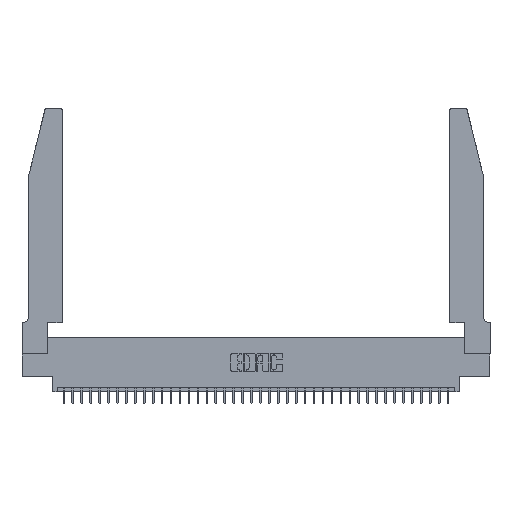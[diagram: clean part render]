
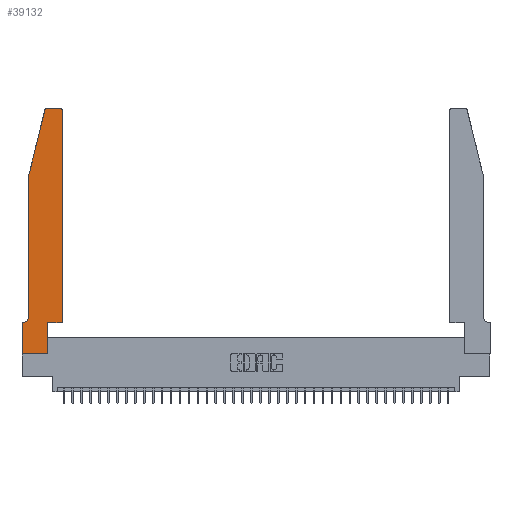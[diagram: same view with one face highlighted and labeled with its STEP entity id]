
A CAD part, top view. The second image highlights one B-rep face of the part: STEP entity #39132.
In plain terms, the highlighted planar face has unit normal (0, 0, 1).
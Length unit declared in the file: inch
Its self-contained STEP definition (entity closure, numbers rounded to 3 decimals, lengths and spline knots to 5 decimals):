
#134 = VERTEX_POINT ( 'NONE', #5959 ) ;
#214 = LINE ( 'NONE', #12319, #29151 ) ;
#238 = CARTESIAN_POINT ( 'NONE',  ( 0.4505, 0.35, 0.37 ) ) ;
#359 = ORIENTED_EDGE ( 'NONE', *, *, #4177, .T. ) ;
#450 = ORIENTED_EDGE ( 'NONE', *, *, #17238, .T. ) ;
#1116 = VECTOR ( 'NONE', #9375, 39.37008 ) ;
#1347 = DIRECTION ( 'NONE',  ( 1., 0., 0. ) ) ;
#1585 = AXIS2_PLACEMENT_3D ( 'NONE', #24656, #33210, #23868 ) ;
#1913 = CARTESIAN_POINT ( 'NONE',  ( 0.2865, 0.35, 0.37 ) ) ;
#2260 = DIRECTION ( 'NONE',  ( -1., 0., 0. ) ) ;
#3173 = LINE ( 'NONE', #27199, #30112 ) ;
#4101 = DIRECTION ( 'NONE',  ( 0., 0., 1. ) ) ;
#4177 = EDGE_CURVE ( 'NONE', #26298, #17205, #36339, .T. ) ;
#4184 = LINE ( 'NONE', #6785, #25889 ) ;
#4280 = CARTESIAN_POINT ( 'NONE',  ( 0., 0., 0.37 ) ) ;
#4679 = ORIENTED_EDGE ( 'NONE', *, *, #5026, .T. ) ;
#4870 = CARTESIAN_POINT ( 'NONE',  ( 0.25487, 2.72718, 0.37 ) ) ;
#5026 = EDGE_CURVE ( 'NONE', #14524, #21064, #29655, .T. ) ;
#5142 = EDGE_CURVE ( 'NONE', #17487, #14524, #12159, .T. ) ;
#5277 = ORIENTED_EDGE ( 'NONE', *, *, #14382, .T. ) ;
#5580 = VECTOR ( 'NONE', #23078, 39.37008 ) ;
#5959 = CARTESIAN_POINT ( 'NONE',  ( 0.2865, 0., 0.37 ) ) ;
#6634 = EDGE_CURVE ( 'NONE', #17205, #21203, #7933, .T. ) ;
#6785 = CARTESIAN_POINT ( 'NONE',  ( 0.2865, 0.35, 0.37 ) ) ;
#7209 = VECTOR ( 'NONE', #10665, 39.37008 ) ;
#7933 = LINE ( 'NONE', #16682, #13136 ) ;
#8390 = CARTESIAN_POINT ( 'NONE',  ( 0., 0.35, 0.37 ) ) ;
#8441 = EDGE_LOOP ( 'NONE', ( #31779, #32992, #359, #36235, #29790, #37587, #19989, #450, #5277, #27874, #4679, #32138 ) ) ;
#9365 = EDGE_CURVE ( 'NONE', #35133, #26298, #33944, .T. ) ;
#9375 = DIRECTION ( 'NONE',  ( 1., 0., 0. ) ) ;
#9618 = DIRECTION ( 'NONE',  ( 0., 0., -1. ) ) ;
#10665 = DIRECTION ( 'NONE',  ( -1., 0., 0. ) ) ;
#10733 = DIRECTION ( 'NONE',  ( 0., 0., 1. ) ) ;
#11604 = LINE ( 'NONE', #24296, #25306 ) ;
#12159 = LINE ( 'NONE', #238, #1116 ) ;
#12319 = CARTESIAN_POINT ( 'NONE',  ( 0., 0., 0.37 ) ) ;
#12712 = VERTEX_POINT ( 'NONE', #8390 ) ;
#13136 = VECTOR ( 'NONE', #25631, 39.37008 ) ;
#13254 = LINE ( 'NONE', #25562, #7209 ) ;
#13689 = CARTESIAN_POINT ( 'NONE',  ( 0.284, 2.75, 0.37 ) ) ;
#14382 = EDGE_CURVE ( 'NONE', #134, #17487, #4184, .T. ) ;
#14524 = VERTEX_POINT ( 'NONE', #32408 ) ;
#14964 = DIRECTION ( 'NONE',  ( 0., -1., 0. ) ) ;
#15475 = CARTESIAN_POINT ( 'NONE',  ( 0.4505, 2.72, 0.37 ) ) ;
#15650 = VECTOR ( 'NONE', #20848, 39.37008 ) ;
#15652 = CARTESIAN_POINT ( 'NONE',  ( 0.0755, 2., 0.37 ) ) ;
#16485 = DIRECTION ( 'NONE',  ( 1., 0., 0. ) ) ;
#16682 = CARTESIAN_POINT ( 'NONE',  ( 0.0755, 2., 0.37 ) ) ;
#17205 = VERTEX_POINT ( 'NONE', #17900 ) ;
#17238 = EDGE_CURVE ( 'NONE', #19877, #134, #214, .T. ) ;
#17487 = VERTEX_POINT ( 'NONE', #1913 ) ;
#17886 = VERTEX_POINT ( 'NONE', #29994 ) ;
#17900 = CARTESIAN_POINT ( 'NONE',  ( 0.0755, 2., 0.37 ) ) ;
#18156 = CARTESIAN_POINT ( 'NONE',  ( 0.0055, 0.42, 0.37 ) ) ;
#18944 = EDGE_CURVE ( 'NONE', #21203, #17886, #27215, .T. ) ;
#19877 = VERTEX_POINT ( 'NONE', #4280 ) ;
#19989 = ORIENTED_EDGE ( 'NONE', *, *, #30989, .T. ) ;
#20848 = DIRECTION ( 'NONE',  ( -0.239, -0.971, 0. ) ) ;
#21064 = VERTEX_POINT ( 'NONE', #15475 ) ;
#21203 = VERTEX_POINT ( 'NONE', #31942 ) ;
#21972 = FACE_OUTER_BOUND ( 'NONE', #8441, .T. ) ;
#23078 = DIRECTION ( 'NONE',  ( 0., 1., 0. ) ) ;
#23868 = DIRECTION ( 'NONE',  ( 1., 0., 0. ) ) ;
#24296 = CARTESIAN_POINT ( 'NONE',  ( 0., 0., 0.37 ) ) ;
#24656 = CARTESIAN_POINT ( 'NONE',  ( 0.284, 2.72, 0.37 ) ) ;
#25306 = VECTOR ( 'NONE', #14964, 39.37008 ) ;
#25562 = CARTESIAN_POINT ( 'NONE',  ( 0.2605, 2.75, 0.37 ) ) ;
#25631 = DIRECTION ( 'NONE',  ( 0., -1., 0. ) ) ;
#25889 = VECTOR ( 'NONE', #33647, 39.37008 ) ;
#26032 = CARTESIAN_POINT ( 'NONE',  ( 0.4205, 2.72, 0.37 ) ) ;
#26298 = VERTEX_POINT ( 'NONE', #4870 ) ;
#26694 = AXIS2_PLACEMENT_3D ( 'NONE', #26032, #10733, #16485 ) ;
#27199 = CARTESIAN_POINT ( 'NONE',  ( 0.0755, 0.35, 0.37 ) ) ;
#27215 = CIRCLE ( 'NONE', #33587, 0.07 ) ;
#27874 = ORIENTED_EDGE ( 'NONE', *, *, #5142, .T. ) ;
#28559 = CARTESIAN_POINT ( 'NONE',  ( 0., 0.35, 0.37 ) ) ;
#29078 = CARTESIAN_POINT ( 'NONE',  ( 0.4505, 0.35, 0.37 ) ) ;
#29151 = VECTOR ( 'NONE', #36187, 39.37008 ) ;
#29404 = AXIS2_PLACEMENT_3D ( 'NONE', #28559, #4101, #1347 ) ;
#29655 = LINE ( 'NONE', #29078, #5580 ) ;
#29790 = ORIENTED_EDGE ( 'NONE', *, *, #18944, .T. ) ;
#29994 = CARTESIAN_POINT ( 'NONE',  ( 0.0055, 0.35, 0.37 ) ) ;
#30112 = VECTOR ( 'NONE', #2260, 39.37008 ) ;
#30804 = CARTESIAN_POINT ( 'NONE',  ( 0.4205, 2.75, 0.37 ) ) ;
#30989 = EDGE_CURVE ( 'NONE', #12712, #19877, #11604, .T. ) ;
#31779 = ORIENTED_EDGE ( 'NONE', *, *, #37856, .T. ) ;
#31942 = CARTESIAN_POINT ( 'NONE',  ( 0.0755, 0.42, 0.37 ) ) ;
#32138 = ORIENTED_EDGE ( 'NONE', *, *, #33020, .T. ) ;
#32408 = CARTESIAN_POINT ( 'NONE',  ( 0.4505, 0.35, 0.37 ) ) ;
#32881 = VERTEX_POINT ( 'NONE', #30804 ) ;
#32992 = ORIENTED_EDGE ( 'NONE', *, *, #9365, .T. ) ;
#33020 = EDGE_CURVE ( 'NONE', #21064, #32881, #37494, .T. ) ;
#33210 = DIRECTION ( 'NONE',  ( 0., 0., 1. ) ) ;
#33587 = AXIS2_PLACEMENT_3D ( 'NONE', #18156, #9618, #33858 ) ;
#33647 = DIRECTION ( 'NONE',  ( 0., 1., 0. ) ) ;
#33858 = DIRECTION ( 'NONE',  ( -1., 0., 0. ) ) ;
#33944 = CIRCLE ( 'NONE', #1585, 0.03 ) ;
#34136 = PLANE ( 'NONE',  #29404 ) ;
#35133 = VERTEX_POINT ( 'NONE', #13689 ) ;
#36187 = DIRECTION ( 'NONE',  ( 1., 0., 0. ) ) ;
#36235 = ORIENTED_EDGE ( 'NONE', *, *, #6634, .T. ) ;
#36339 = LINE ( 'NONE', #15652, #15650 ) ;
#37494 = CIRCLE ( 'NONE', #26694, 0.03 ) ;
#37587 = ORIENTED_EDGE ( 'NONE', *, *, #39000, .T. ) ;
#37856 = EDGE_CURVE ( 'NONE', #32881, #35133, #13254, .T. ) ;
#39000 = EDGE_CURVE ( 'NONE', #17886, #12712, #3173, .T. ) ;
#39132 = ADVANCED_FACE ( 'NONE', ( #21972 ), #34136, .T. ) ;
